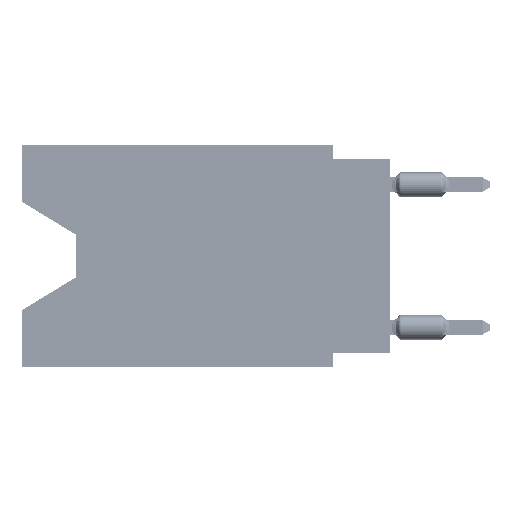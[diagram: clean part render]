
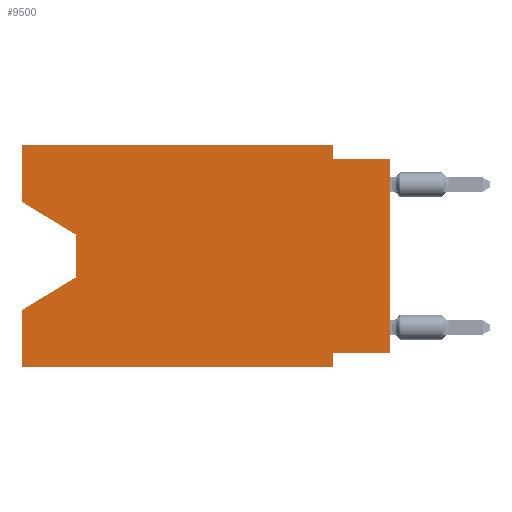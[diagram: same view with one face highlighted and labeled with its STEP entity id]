
A CAD part, left-side view. The second image highlights one B-rep face of the part: STEP entity #9500.
In plain terms, the highlighted planar face has unit normal (-1, 0, 0).
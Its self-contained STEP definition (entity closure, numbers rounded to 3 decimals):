
#361 = EDGE_CURVE ( 'NONE', #32900, #29126, #33483, .T. ) ;
#516 = LINE ( 'NONE', #41515, #34059 ) ;
#1717 = CARTESIAN_POINT ( 'NONE',  ( 0., 16.383, -7.36 ) ) ;
#1856 = CARTESIAN_POINT ( 'NONE',  ( 0., 2.54, -9.906 ) ) ;
#1940 = PLANE ( 'NONE',  #39404 ) ;
#2181 = CARTESIAN_POINT ( 'NONE',  ( 0., 2.54, -9.906 ) ) ;
#2328 = ORIENTED_EDGE ( 'NONE', *, *, #65517, .T. ) ;
#4233 = DIRECTION ( 'NONE',  ( 0., -1., 0. ) ) ;
#4389 = VECTOR ( 'NONE', #66095, 1000. ) ;
#5040 = ORIENTED_EDGE ( 'NONE', *, *, #10986, .T. ) ;
#6316 = FACE_OUTER_BOUND ( 'NONE', #50082, .T. ) ;
#6724 = CARTESIAN_POINT ( 'NONE',  ( 0., 16.383, -9.906 ) ) ;
#7608 = DIRECTION ( 'NONE',  ( 0., -0.855, -0.519 ) ) ;
#9171 = VERTEX_POINT ( 'NONE', #33597 ) ;
#9349 = VERTEX_POINT ( 'NONE', #25839 ) ;
#9500 = ADVANCED_FACE ( 'NONE', ( #6316 ), #1940, .F. ) ;
#10326 = VECTOR ( 'NONE', #15038, 1000. ) ;
#10539 = CARTESIAN_POINT ( 'NONE',  ( 0., 0., -9.271 ) ) ;
#10986 = EDGE_CURVE ( 'NONE', #29126, #49582, #40218, .T. ) ;
#14079 = EDGE_CURVE ( 'NONE', #32235, #19714, #47865, .T. ) ;
#14306 = CARTESIAN_POINT ( 'NONE',  ( 0., 0., -0.635 ) ) ;
#15038 = DIRECTION ( 'NONE',  ( 0., 0., 1. ) ) ;
#15785 = ORIENTED_EDGE ( 'NONE', *, *, #19594, .F. ) ;
#15961 = EDGE_CURVE ( 'NONE', #27873, #19714, #52423, .T. ) ;
#16818 = DIRECTION ( 'NONE',  ( 0., -1., 0. ) ) ;
#18310 = DIRECTION ( 'NONE',  ( 0., 0., -1. ) ) ;
#18509 = CARTESIAN_POINT ( 'NONE',  ( 0., 16.383, 0. ) ) ;
#18697 = VERTEX_POINT ( 'NONE', #25332 ) ;
#18705 = CARTESIAN_POINT ( 'NONE',  ( 0., 0., -0.635 ) ) ;
#18754 = VECTOR ( 'NONE', #16818, 1000. ) ;
#19594 = EDGE_CURVE ( 'NONE', #9349, #9171, #516, .T. ) ;
#19714 = VERTEX_POINT ( 'NONE', #1856 ) ;
#21021 = CARTESIAN_POINT ( 'NONE',  ( 0., 2.54, -0.635 ) ) ;
#22485 = VECTOR ( 'NONE', #31054, 1000. ) ;
#22727 = CARTESIAN_POINT ( 'NONE',  ( 0., 0., 0. ) ) ;
#22887 = LINE ( 'NONE', #59820, #59457 ) ;
#22914 = ORIENTED_EDGE ( 'NONE', *, *, #58738, .F. ) ;
#22957 = VECTOR ( 'NONE', #54280, 1000. ) ;
#23544 = ORIENTED_EDGE ( 'NONE', *, *, #64062, .F. ) ;
#24069 = LINE ( 'NONE', #29131, #49051 ) ;
#24216 = ORIENTED_EDGE ( 'NONE', *, *, #361, .T. ) ;
#24647 = VERTEX_POINT ( 'NONE', #21021 ) ;
#25332 = CARTESIAN_POINT ( 'NONE',  ( 0., 0., -9.271 ) ) ;
#25839 = CARTESIAN_POINT ( 'NONE',  ( 0., 16.383, 0. ) ) ;
#26404 = CARTESIAN_POINT ( 'NONE',  ( 0., 13.97, -4.013 ) ) ;
#26820 = DIRECTION ( 'NONE',  ( 0., 0., -1. ) ) ;
#27873 = VERTEX_POINT ( 'NONE', #62996 ) ;
#29126 = VERTEX_POINT ( 'NONE', #38939 ) ;
#29131 = CARTESIAN_POINT ( 'NONE',  ( 0., 2.54, 0. ) ) ;
#30767 = VERTEX_POINT ( 'NONE', #18705 ) ;
#31054 = DIRECTION ( 'NONE',  ( 0., 1., 0. ) ) ;
#31535 = VECTOR ( 'NONE', #66230, 1000. ) ;
#32235 = VERTEX_POINT ( 'NONE', #66082 ) ;
#32900 = VERTEX_POINT ( 'NONE', #40101 ) ;
#33483 = LINE ( 'NONE', #33810, #42592 ) ;
#33597 = CARTESIAN_POINT ( 'NONE',  ( 0., 2.54, 0. ) ) ;
#33810 = CARTESIAN_POINT ( 'NONE',  ( 0., 16.383, -2.546 ) ) ;
#34059 = VECTOR ( 'NONE', #51266, 1000. ) ;
#38281 = ORIENTED_EDGE ( 'NONE', *, *, #14079, .F. ) ;
#38939 = CARTESIAN_POINT ( 'NONE',  ( 0., 13.97, -4.013 ) ) ;
#39404 = AXIS2_PLACEMENT_3D ( 'NONE', #42253, #52678, #26820 ) ;
#40101 = CARTESIAN_POINT ( 'NONE',  ( 0., 16.383, -2.546 ) ) ;
#40218 = LINE ( 'NONE', #26404, #4389 ) ;
#41515 = CARTESIAN_POINT ( 'NONE',  ( 0., 16.383, 0. ) ) ;
#42253 = CARTESIAN_POINT ( 'NONE',  ( 0., 16.383, 0. ) ) ;
#42592 = VECTOR ( 'NONE', #7608, 1000. ) ;
#43259 = EDGE_CURVE ( 'NONE', #49582, #47668, #22887, .T. ) ;
#43596 = ORIENTED_EDGE ( 'NONE', *, *, #50200, .F. ) ;
#43804 = CARTESIAN_POINT ( 'NONE',  ( 0., 16.383, 0. ) ) ;
#43966 = VECTOR ( 'NONE', #4233, 1000. ) ;
#45704 = LINE ( 'NONE', #43804, #31535 ) ;
#46810 = LINE ( 'NONE', #10539, #22485 ) ;
#47033 = ORIENTED_EDGE ( 'NONE', *, *, #15961, .T. ) ;
#47668 = VERTEX_POINT ( 'NONE', #1717 ) ;
#47767 = EDGE_CURVE ( 'NONE', #27873, #47668, #55697, .T. ) ;
#47865 = LINE ( 'NONE', #2181, #55184 ) ;
#49051 = VECTOR ( 'NONE', #59021, 1000. ) ;
#49582 = VERTEX_POINT ( 'NONE', #50629 ) ;
#50082 = EDGE_LOOP ( 'NONE', ( #24216, #5040, #66047, #64962, #47033, #38281, #43596, #2328, #22914, #54118, #15785, #23544 ) ) ;
#50200 = EDGE_CURVE ( 'NONE', #18697, #32235, #46810, .T. ) ;
#50629 = CARTESIAN_POINT ( 'NONE',  ( 0., 13.97, -5.893 ) ) ;
#51266 = DIRECTION ( 'NONE',  ( 0., -1., 0. ) ) ;
#52423 = LINE ( 'NONE', #6724, #18754 ) ;
#52678 = DIRECTION ( 'NONE',  ( 1., 0., 0. ) ) ;
#54118 = ORIENTED_EDGE ( 'NONE', *, *, #58553, .F. ) ;
#54280 = DIRECTION ( 'NONE',  ( 0., 0., 1. ) ) ;
#55184 = VECTOR ( 'NONE', #18310, 1000. ) ;
#55697 = LINE ( 'NONE', #18509, #10326 ) ;
#58553 = EDGE_CURVE ( 'NONE', #9171, #24647, #24069, .T. ) ;
#58738 = EDGE_CURVE ( 'NONE', #24647, #30767, #61346, .T. ) ;
#59021 = DIRECTION ( 'NONE',  ( 0., 0., -1. ) ) ;
#59318 = LINE ( 'NONE', #22727, #22957 ) ;
#59457 = VECTOR ( 'NONE', #64537, 1000. ) ;
#59820 = CARTESIAN_POINT ( 'NONE',  ( 0., 13.97, -5.893 ) ) ;
#61346 = LINE ( 'NONE', #14306, #43966 ) ;
#62996 = CARTESIAN_POINT ( 'NONE',  ( 0., 16.383, -9.906 ) ) ;
#64062 = EDGE_CURVE ( 'NONE', #32900, #9349, #45704, .T. ) ;
#64537 = DIRECTION ( 'NONE',  ( 0., 0.855, -0.519 ) ) ;
#64962 = ORIENTED_EDGE ( 'NONE', *, *, #47767, .F. ) ;
#65517 = EDGE_CURVE ( 'NONE', #18697, #30767, #59318, .T. ) ;
#66047 = ORIENTED_EDGE ( 'NONE', *, *, #43259, .T. ) ;
#66082 = CARTESIAN_POINT ( 'NONE',  ( 0., 2.54, -9.271 ) ) ;
#66095 = DIRECTION ( 'NONE',  ( 0., 0., -1. ) ) ;
#66230 = DIRECTION ( 'NONE',  ( 0., 0., 1. ) ) ;
